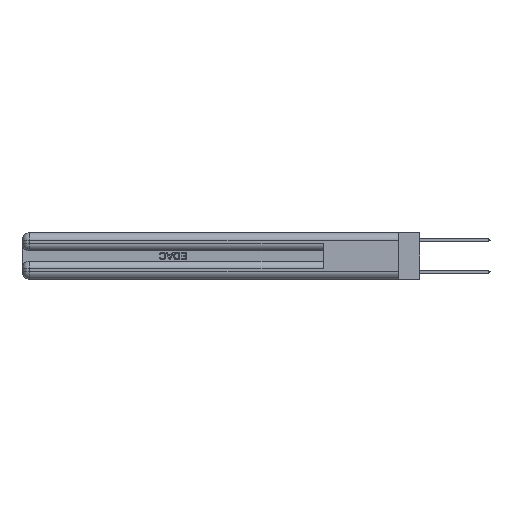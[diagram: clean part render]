
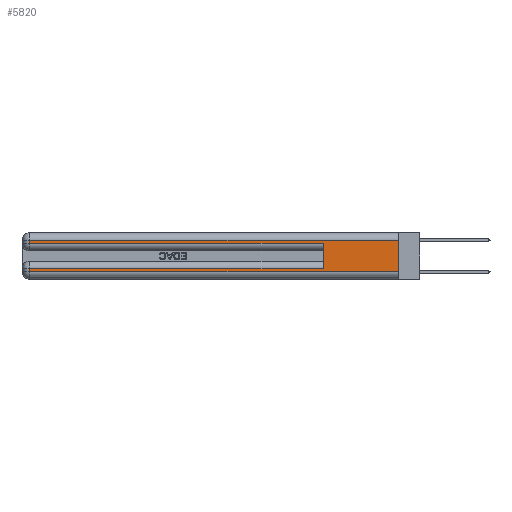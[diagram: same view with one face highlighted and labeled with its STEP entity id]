
A CAD part, left-side view. The second image highlights one B-rep face of the part: STEP entity #5820.
In plain terms, the highlighted planar face has unit normal (-1, 0, 0).
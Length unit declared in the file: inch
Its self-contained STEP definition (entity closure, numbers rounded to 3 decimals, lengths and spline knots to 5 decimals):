
#1445 = CARTESIAN_POINT ( 'NONE',  ( 0., 0., 0.06 ) ) ;
#2228 = VECTOR ( 'NONE', #17723, 39.37008 ) ;
#2622 = DIRECTION ( 'NONE',  ( 0., 0., -1. ) ) ;
#3623 = CARTESIAN_POINT ( 'NONE',  ( 0., 0.6, 0.145 ) ) ;
#3783 = ORIENTED_EDGE ( 'NONE', *, *, #25409, .T. ) ;
#4138 = DIRECTION ( 'NONE',  ( 0., 0., -1. ) ) ;
#4312 = DIRECTION ( 'NONE',  ( 0., -1., 0. ) ) ;
#5484 = VERTEX_POINT ( 'NONE', #33776 ) ;
#5614 = EDGE_CURVE ( 'NONE', #10470, #9454, #7161, .T. ) ;
#5651 = EDGE_CURVE ( 'NONE', #12377, #10470, #15384, .T. ) ;
#5820 = ADVANCED_FACE ( 'NONE', ( #11254 ), #15905, .F. ) ;
#6557 = DIRECTION ( 'NONE',  ( 0., 0., -1. ) ) ;
#6984 = CARTESIAN_POINT ( 'NONE',  ( 0., 2.94, 0.37 ) ) ;
#7161 = LINE ( 'NONE', #1445, #19745 ) ;
#8008 = DIRECTION ( 'NONE',  ( 0., 1., 0. ) ) ;
#9454 = VERTEX_POINT ( 'NONE', #29266 ) ;
#9766 = ORIENTED_EDGE ( 'NONE', *, *, #5614, .T. ) ;
#10470 = VERTEX_POINT ( 'NONE', #31867 ) ;
#11254 = FACE_OUTER_BOUND ( 'NONE', #23626, .T. ) ;
#11569 = LINE ( 'NONE', #32475, #13678 ) ;
#12377 = VERTEX_POINT ( 'NONE', #24225 ) ;
#12386 = VECTOR ( 'NONE', #4138, 39.37008 ) ;
#13499 = EDGE_CURVE ( 'NONE', #21042, #14139, #14147, .T. ) ;
#13513 = CARTESIAN_POINT ( 'NONE',  ( 0., 0., 0.37 ) ) ;
#13678 = VECTOR ( 'NONE', #8008, 39.37008 ) ;
#13683 = CARTESIAN_POINT ( 'NONE',  ( 0., 0.6, 0.285 ) ) ;
#13820 = LINE ( 'NONE', #24687, #2228 ) ;
#14139 = VERTEX_POINT ( 'NONE', #13683 ) ;
#14147 = LINE ( 'NONE', #28410, #23243 ) ;
#14525 = LINE ( 'NONE', #3623, #21978 ) ;
#15384 = LINE ( 'NONE', #6984, #12386 ) ;
#15905 = PLANE ( 'NONE',  #26042 ) ;
#15908 = ORIENTED_EDGE ( 'NONE', *, *, #19712, .F. ) ;
#16054 = CARTESIAN_POINT ( 'NONE',  ( 0., 2.94, 0.285 ) ) ;
#16153 = EDGE_CURVE ( 'NONE', #25302, #5484, #11569, .T. ) ;
#16988 = DIRECTION ( 'NONE',  ( 0., -1., 0. ) ) ;
#17520 = EDGE_CURVE ( 'NONE', #5484, #21042, #20315, .T. ) ;
#17723 = DIRECTION ( 'NONE',  ( 0., 1., 0. ) ) ;
#18621 = ORIENTED_EDGE ( 'NONE', *, *, #13499, .T. ) ;
#18659 = VERTEX_POINT ( 'NONE', #32844 ) ;
#19342 = CARTESIAN_POINT ( 'NONE',  ( 0., 0., 0.31 ) ) ;
#19712 = EDGE_CURVE ( 'NONE', #18659, #14139, #14525, .T. ) ;
#19745 = VECTOR ( 'NONE', #4312, 39.37008 ) ;
#20315 = LINE ( 'NONE', #31029, #22525 ) ;
#20364 = ORIENTED_EDGE ( 'NONE', *, *, #5651, .T. ) ;
#21042 = VERTEX_POINT ( 'NONE', #16054 ) ;
#21344 = LINE ( 'NONE', #13513, #21640 ) ;
#21640 = VECTOR ( 'NONE', #2622, 39.37008 ) ;
#21978 = VECTOR ( 'NONE', #25576, 39.37008 ) ;
#22525 = VECTOR ( 'NONE', #6557, 39.37008 ) ;
#23243 = VECTOR ( 'NONE', #16988, 39.37008 ) ;
#23626 = EDGE_LOOP ( 'NONE', ( #24649, #24532, #23862, #18621, #15908, #3783, #20364, #9766 ) ) ;
#23862 = ORIENTED_EDGE ( 'NONE', *, *, #17520, .T. ) ;
#24225 = CARTESIAN_POINT ( 'NONE',  ( 0., 2.94, 0.085 ) ) ;
#24532 = ORIENTED_EDGE ( 'NONE', *, *, #16153, .T. ) ;
#24649 = ORIENTED_EDGE ( 'NONE', *, *, #24676, .F. ) ;
#24676 = EDGE_CURVE ( 'NONE', #25302, #9454, #21344, .T. ) ;
#24687 = CARTESIAN_POINT ( 'NONE',  ( 0., 0., 0.085 ) ) ;
#25302 = VERTEX_POINT ( 'NONE', #19342 ) ;
#25409 = EDGE_CURVE ( 'NONE', #18659, #12377, #13820, .T. ) ;
#25576 = DIRECTION ( 'NONE',  ( 0., 0., 1. ) ) ;
#26042 = AXIS2_PLACEMENT_3D ( 'NONE', #26777, #30172, #26948 ) ;
#26777 = CARTESIAN_POINT ( 'NONE',  ( 0., 0., 0.37 ) ) ;
#26948 = DIRECTION ( 'NONE',  ( 0., 0., -1. ) ) ;
#28410 = CARTESIAN_POINT ( 'NONE',  ( 0., 0., 0.285 ) ) ;
#29266 = CARTESIAN_POINT ( 'NONE',  ( 0., 0., 0.06 ) ) ;
#30172 = DIRECTION ( 'NONE',  ( 1., 0., 0. ) ) ;
#31029 = CARTESIAN_POINT ( 'NONE',  ( 0., 2.94, 0.37 ) ) ;
#31867 = CARTESIAN_POINT ( 'NONE',  ( 0., 2.94, 0.06 ) ) ;
#32475 = CARTESIAN_POINT ( 'NONE',  ( 0., 0., 0.31 ) ) ;
#32844 = CARTESIAN_POINT ( 'NONE',  ( 0., 0.6, 0.085 ) ) ;
#33776 = CARTESIAN_POINT ( 'NONE',  ( 0., 2.94, 0.31 ) ) ;
